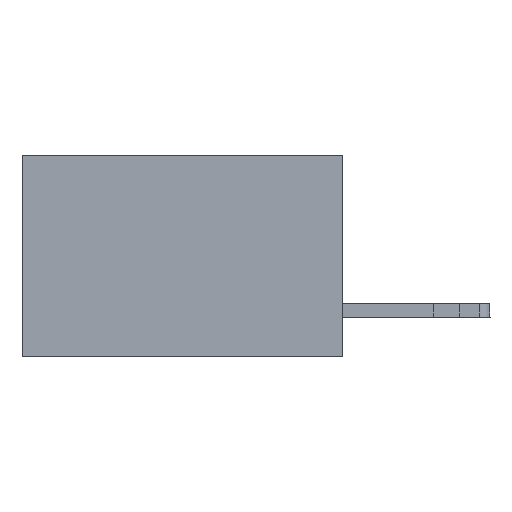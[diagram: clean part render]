
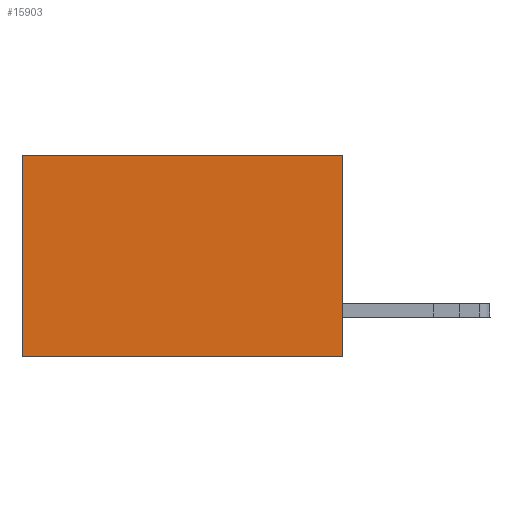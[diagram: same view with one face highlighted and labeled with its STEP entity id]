
A CAD part, left-side view. The second image highlights one B-rep face of the part: STEP entity #15903.
In plain terms, the highlighted planar face has unit normal (-1, 0, 0).
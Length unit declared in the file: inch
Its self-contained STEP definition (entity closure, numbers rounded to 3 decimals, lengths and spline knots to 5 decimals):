
#215 = CARTESIAN_POINT ( 'NONE',  ( 0.277, 0.59, -0.37 ) ) ;
#265 = VERTEX_POINT ( 'NONE', #2424 ) ;
#1049 = ORIENTED_EDGE ( 'NONE', *, *, #9192, .T. ) ;
#1118 = DIRECTION ( 'NONE',  ( 0., 1., 0. ) ) ;
#1305 = CARTESIAN_POINT ( 'NONE',  ( 0.277, 0., -0.37 ) ) ;
#1538 = DIRECTION ( 'NONE',  ( 1., 0., 0. ) ) ;
#2367 = VERTEX_POINT ( 'NONE', #3564 ) ;
#2424 = CARTESIAN_POINT ( 'NONE',  ( 0.277, 0., -0.37 ) ) ;
#2573 = VECTOR ( 'NONE', #17063, 39.37008 ) ;
#2590 = LINE ( 'NONE', #16831, #7113 ) ;
#2946 = CARTESIAN_POINT ( 'NONE',  ( 0.277, 0.59, -0.37 ) ) ;
#2981 = DIRECTION ( 'NONE',  ( 0., 0., -1. ) ) ;
#3564 = CARTESIAN_POINT ( 'NONE',  ( 0.277, 0., 0. ) ) ;
#3870 = CARTESIAN_POINT ( 'NONE',  ( 0.277, 0., -0.37 ) ) ;
#4182 = LINE ( 'NONE', #3870, #2573 ) ;
#7113 = VECTOR ( 'NONE', #1118, 39.37008 ) ;
#7403 = VECTOR ( 'NONE', #2981, 39.37008 ) ;
#7959 = FACE_OUTER_BOUND ( 'NONE', #20741, .T. ) ;
#9192 = EDGE_CURVE ( 'NONE', #18701, #17722, #17106, .T. ) ;
#11984 = EDGE_CURVE ( 'NONE', #265, #17722, #4182, .T. ) ;
#12596 = LINE ( 'NONE', #1305, #7403 ) ;
#12815 = DIRECTION ( 'NONE',  ( 0., 0., -1. ) ) ;
#13552 = ORIENTED_EDGE ( 'NONE', *, *, #18480, .T. ) ;
#13990 = VECTOR ( 'NONE', #20493, 39.37008 ) ;
#14402 = PLANE ( 'NONE',  #20199 ) ;
#14433 = ORIENTED_EDGE ( 'NONE', *, *, #11984, .F. ) ;
#15605 = ORIENTED_EDGE ( 'NONE', *, *, #17157, .F. ) ;
#15903 = ADVANCED_FACE ( 'NONE', ( #7959 ), #14402, .F. ) ;
#16831 = CARTESIAN_POINT ( 'NONE',  ( 0.277, 0., 0. ) ) ;
#17063 = DIRECTION ( 'NONE',  ( 0., 1., 0. ) ) ;
#17106 = LINE ( 'NONE', #2946, #13990 ) ;
#17157 = EDGE_CURVE ( 'NONE', #2367, #265, #12596, .T. ) ;
#17359 = CARTESIAN_POINT ( 'NONE',  ( 0.277, 0.59, 0. ) ) ;
#17722 = VERTEX_POINT ( 'NONE', #215 ) ;
#18480 = EDGE_CURVE ( 'NONE', #2367, #18701, #2590, .T. ) ;
#18701 = VERTEX_POINT ( 'NONE', #17359 ) ;
#20199 = AXIS2_PLACEMENT_3D ( 'NONE', #20859, #1538, #12815 ) ;
#20493 = DIRECTION ( 'NONE',  ( 0., 0., -1. ) ) ;
#20741 = EDGE_LOOP ( 'NONE', ( #1049, #14433, #15605, #13552 ) ) ;
#20859 = CARTESIAN_POINT ( 'NONE',  ( 0.277, 0., -0.37 ) ) ;
